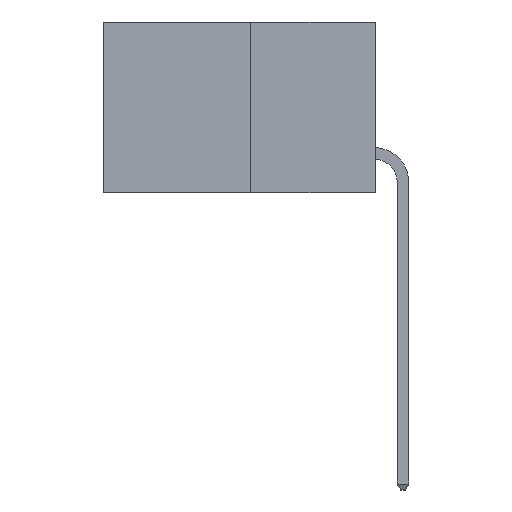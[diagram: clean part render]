
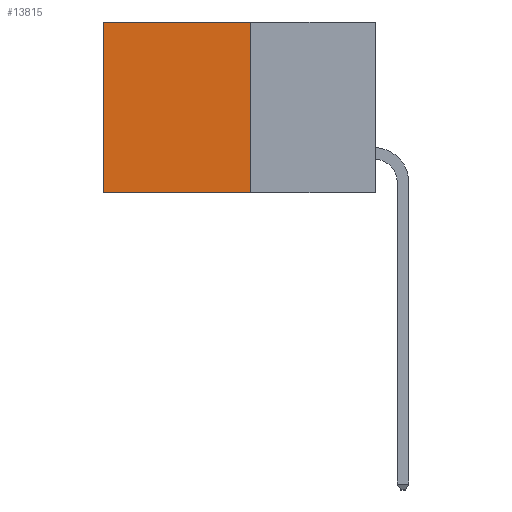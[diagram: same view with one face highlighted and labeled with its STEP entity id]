
A CAD part, left-side view. The second image highlights one B-rep face of the part: STEP entity #13815.
In plain terms, the highlighted planar face has unit normal (-1, 0, 0).
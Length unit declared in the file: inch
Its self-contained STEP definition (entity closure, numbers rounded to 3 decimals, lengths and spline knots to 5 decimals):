
#23 = ORIENTED_EDGE ( 'NONE', *, *, #4059, .T. ) ;
#389 = VERTEX_POINT ( 'NONE', #3554 ) ;
#493 = LINE ( 'NONE', #19071, #12687 ) ;
#596 = CARTESIAN_POINT ( 'NONE',  ( 0.277, 0.27, -0.37 ) ) ;
#888 = VECTOR ( 'NONE', #16478, 39.37008 ) ;
#972 = VERTEX_POINT ( 'NONE', #596 ) ;
#2311 = VECTOR ( 'NONE', #7877, 39.37008 ) ;
#2435 = CARTESIAN_POINT ( 'NONE',  ( 0.277, 0.59, 0. ) ) ;
#2488 = VERTEX_POINT ( 'NONE', #2435 ) ;
#2550 = EDGE_CURVE ( 'NONE', #11408, #972, #4133, .T. ) ;
#2714 = DIRECTION ( 'NONE',  ( 1., 0., 0. ) ) ;
#3252 = CARTESIAN_POINT ( 'NONE',  ( 0.277, 0.27, -0.37 ) ) ;
#3554 = CARTESIAN_POINT ( 'NONE',  ( 0.277, 0.59, -0.37 ) ) ;
#4059 = EDGE_CURVE ( 'NONE', #2488, #389, #493, .T. ) ;
#4133 = LINE ( 'NONE', #3252, #16101 ) ;
#5026 = FACE_OUTER_BOUND ( 'NONE', #10802, .T. ) ;
#5581 = DIRECTION ( 'NONE',  ( 0., 0., -1. ) ) ;
#7877 = DIRECTION ( 'NONE',  ( 0., 1., 0. ) ) ;
#8494 = ORIENTED_EDGE ( 'NONE', *, *, #2550, .F. ) ;
#10621 = DIRECTION ( 'NONE',  ( 0., 0., -1. ) ) ;
#10802 = EDGE_LOOP ( 'NONE', ( #23, #16124, #8494, #14511 ) ) ;
#11408 = VERTEX_POINT ( 'NONE', #16980 ) ;
#12118 = EDGE_CURVE ( 'NONE', #972, #389, #17990, .T. ) ;
#12205 = CARTESIAN_POINT ( 'NONE',  ( 0.277, 0.27, -0.37 ) ) ;
#12687 = VECTOR ( 'NONE', #10621, 39.37008 ) ;
#13540 = LINE ( 'NONE', #14937, #888 ) ;
#13739 = DIRECTION ( 'NONE',  ( 0., 0., -1. ) ) ;
#13815 = ADVANCED_FACE ( 'NONE', ( #5026 ), #15212, .F. ) ;
#14511 = ORIENTED_EDGE ( 'NONE', *, *, #18841, .T. ) ;
#14937 = CARTESIAN_POINT ( 'NONE',  ( 0.277, 0.27, 0. ) ) ;
#15212 = PLANE ( 'NONE',  #16479 ) ;
#16101 = VECTOR ( 'NONE', #5581, 39.37008 ) ;
#16124 = ORIENTED_EDGE ( 'NONE', *, *, #12118, .F. ) ;
#16478 = DIRECTION ( 'NONE',  ( 0., 1., 0. ) ) ;
#16479 = AXIS2_PLACEMENT_3D ( 'NONE', #12205, #2714, #13739 ) ;
#16980 = CARTESIAN_POINT ( 'NONE',  ( 0.277, 0.27, 0. ) ) ;
#17990 = LINE ( 'NONE', #18651, #2311 ) ;
#18651 = CARTESIAN_POINT ( 'NONE',  ( 0.277, 0.27, -0.37 ) ) ;
#18841 = EDGE_CURVE ( 'NONE', #11408, #2488, #13540, .T. ) ;
#19071 = CARTESIAN_POINT ( 'NONE',  ( 0.277, 0.59, -0.37 ) ) ;
